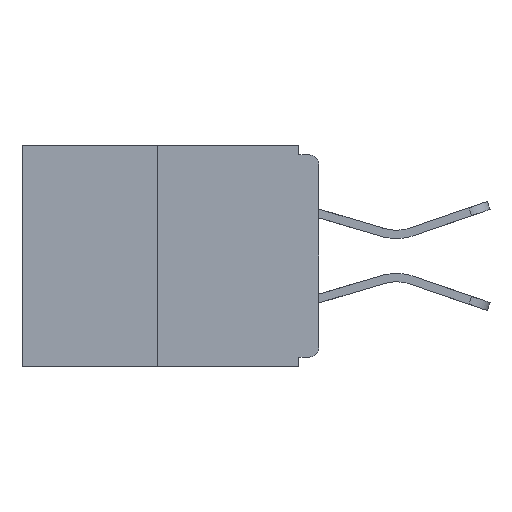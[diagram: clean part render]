
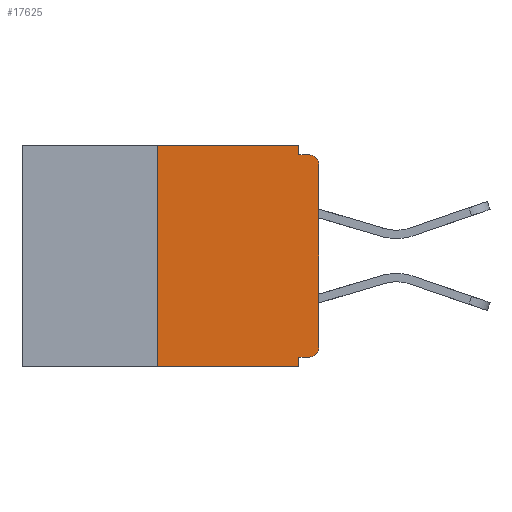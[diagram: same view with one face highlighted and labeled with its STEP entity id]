
A CAD part, left-side view. The second image highlights one B-rep face of the part: STEP entity #17625.
In plain terms, the highlighted planar face has unit normal (-1, 0, 0).
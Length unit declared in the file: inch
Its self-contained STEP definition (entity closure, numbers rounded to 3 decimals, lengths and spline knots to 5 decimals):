
#193 = VECTOR ( 'NONE', #14481, 39.37008 ) ;
#308 = DIRECTION ( 'NONE',  ( 0., 0., -1. ) ) ;
#543 = EDGE_CURVE ( 'NONE', #5200, #4194, #3123, .T. ) ;
#888 = EDGE_CURVE ( 'NONE', #13235, #17424, #23163, .T. ) ;
#1353 = CARTESIAN_POINT ( 'NONE',  ( 0., 0.031, 0. ) ) ;
#1658 = CARTESIAN_POINT ( 'NONE',  ( 0., 0.46, 0. ) ) ;
#2864 = CIRCLE ( 'NONE', #9612, 0.015 ) ;
#3123 = LINE ( 'NONE', #16304, #193 ) ;
#3310 = ORIENTED_EDGE ( 'NONE', *, *, #22976, .F. ) ;
#4194 = VERTEX_POINT ( 'NONE', #15038 ) ;
#4618 = CARTESIAN_POINT ( 'NONE',  ( 0., 0., 0. ) ) ;
#5200 = VERTEX_POINT ( 'NONE', #6665 ) ;
#5309 = VECTOR ( 'NONE', #15699, 39.37008 ) ;
#5706 = EDGE_CURVE ( 'NONE', #8212, #19450, #11725, .T. ) ;
#6344 = EDGE_CURVE ( 'NONE', #8212, #4194, #7748, .T. ) ;
#6628 = CARTESIAN_POINT ( 'NONE',  ( 0., 0., -0.328 ) ) ;
#6665 = CARTESIAN_POINT ( 'NONE',  ( 0., 0.031, -0.328 ) ) ;
#7054 = VECTOR ( 'NONE', #19556, 39.37008 ) ;
#7323 = EDGE_CURVE ( 'NONE', #19450, #19674, #19778, .T. ) ;
#7455 = CARTESIAN_POINT ( 'NONE',  ( 0., 0.031, -0.015 ) ) ;
#7739 = AXIS2_PLACEMENT_3D ( 'NONE', #13149, #18958, #15122 ) ;
#7748 = LINE ( 'NONE', #9975, #16897 ) ;
#7854 = ORIENTED_EDGE ( 'NONE', *, *, #6344, .T. ) ;
#8212 = VERTEX_POINT ( 'NONE', #15849 ) ;
#8448 = EDGE_CURVE ( 'NONE', #22660, #9009, #17925, .T. ) ;
#8456 = ORIENTED_EDGE ( 'NONE', *, *, #17105, .T. ) ;
#8824 = EDGE_CURVE ( 'NONE', #12329, #22660, #21196, .T. ) ;
#9009 = VERTEX_POINT ( 'NONE', #17903 ) ;
#9612 = AXIS2_PLACEMENT_3D ( 'NONE', #17090, #15550, #308 ) ;
#9975 = CARTESIAN_POINT ( 'NONE',  ( 0., 0.46, -0.343 ) ) ;
#10385 = DIRECTION ( 'NONE',  ( 0., 1., 0. ) ) ;
#10812 = DIRECTION ( 'NONE',  ( 0., -1., 0. ) ) ;
#10922 = ORIENTED_EDGE ( 'NONE', *, *, #7323, .F. ) ;
#11391 = FACE_OUTER_BOUND ( 'NONE', #20307, .T. ) ;
#11452 = PLANE ( 'NONE',  #7739 ) ;
#11725 = LINE ( 'NONE', #23120, #7054 ) ;
#11964 = DIRECTION ( 'NONE',  ( 0., -1., 0. ) ) ;
#12041 = ORIENTED_EDGE ( 'NONE', *, *, #543, .F. ) ;
#12329 = VERTEX_POINT ( 'NONE', #19905 ) ;
#13149 = CARTESIAN_POINT ( 'NONE',  ( 0., 0.46, 0. ) ) ;
#13235 = VERTEX_POINT ( 'NONE', #7455 ) ;
#14386 = CARTESIAN_POINT ( 'NONE',  ( 0., 0.015, -0.015 ) ) ;
#14481 = DIRECTION ( 'NONE',  ( 0., 0., -1. ) ) ;
#15038 = CARTESIAN_POINT ( 'NONE',  ( 0., 0.031, -0.343 ) ) ;
#15122 = DIRECTION ( 'NONE',  ( 0., 0., -1. ) ) ;
#15478 = ORIENTED_EDGE ( 'NONE', *, *, #8448, .T. ) ;
#15550 = DIRECTION ( 'NONE',  ( -1., 0., 0. ) ) ;
#15699 = DIRECTION ( 'NONE',  ( 0., 0., -1. ) ) ;
#15849 = CARTESIAN_POINT ( 'NONE',  ( 0., 0.25, -0.343 ) ) ;
#15937 = CARTESIAN_POINT ( 'NONE',  ( 0., 0.031, 0. ) ) ;
#16105 = VECTOR ( 'NONE', #11964, 39.37008 ) ;
#16304 = CARTESIAN_POINT ( 'NONE',  ( 0., 0.031, -0.343 ) ) ;
#16751 = LINE ( 'NONE', #15937, #5309 ) ;
#16897 = VECTOR ( 'NONE', #21461, 39.37008 ) ;
#17090 = CARTESIAN_POINT ( 'NONE',  ( 0., 0.015, -0.03 ) ) ;
#17105 = EDGE_CURVE ( 'NONE', #9009, #17424, #2864, .T. ) ;
#17332 = CARTESIAN_POINT ( 'NONE',  ( 0., 0.015, -0.313 ) ) ;
#17413 = DIRECTION ( 'NONE',  ( -1., 0., 0. ) ) ;
#17424 = VERTEX_POINT ( 'NONE', #14386 ) ;
#17602 = ORIENTED_EDGE ( 'NONE', *, *, #888, .F. ) ;
#17625 = ADVANCED_FACE ( 'NONE', ( #11391 ), #11452, .F. ) ;
#17903 = CARTESIAN_POINT ( 'NONE',  ( 0., 0., -0.03 ) ) ;
#17925 = LINE ( 'NONE', #4618, #18529 ) ;
#18529 = VECTOR ( 'NONE', #19691, 39.37008 ) ;
#18958 = DIRECTION ( 'NONE',  ( 1., 0., 0. ) ) ;
#19177 = VECTOR ( 'NONE', #10812, 39.37008 ) ;
#19237 = DIRECTION ( 'NONE',  ( 0., 0., -1. ) ) ;
#19450 = VERTEX_POINT ( 'NONE', #23061 ) ;
#19556 = DIRECTION ( 'NONE',  ( 0., 0., 1. ) ) ;
#19674 = VERTEX_POINT ( 'NONE', #1353 ) ;
#19691 = DIRECTION ( 'NONE',  ( 0., 0., 1. ) ) ;
#19778 = LINE ( 'NONE', #1658, #19177 ) ;
#19792 = CARTESIAN_POINT ( 'NONE',  ( 0., 0., -0.015 ) ) ;
#19905 = CARTESIAN_POINT ( 'NONE',  ( 0., 0.015, -0.328 ) ) ;
#20307 = EDGE_LOOP ( 'NONE', ( #10922, #22614, #7854, #12041, #23509, #21224, #15478, #8456, #17602, #3310 ) ) ;
#20331 = EDGE_CURVE ( 'NONE', #12329, #5200, #22822, .T. ) ;
#21196 = CIRCLE ( 'NONE', #21814, 0.015 ) ;
#21224 = ORIENTED_EDGE ( 'NONE', *, *, #8824, .T. ) ;
#21461 = DIRECTION ( 'NONE',  ( 0., -1., 0. ) ) ;
#21814 = AXIS2_PLACEMENT_3D ( 'NONE', #17332, #17413, #19237 ) ;
#22298 = CARTESIAN_POINT ( 'NONE',  ( 0., 0., -0.313 ) ) ;
#22614 = ORIENTED_EDGE ( 'NONE', *, *, #5706, .F. ) ;
#22660 = VERTEX_POINT ( 'NONE', #22298 ) ;
#22822 = LINE ( 'NONE', #6628, #23415 ) ;
#22976 = EDGE_CURVE ( 'NONE', #19674, #13235, #16751, .T. ) ;
#23061 = CARTESIAN_POINT ( 'NONE',  ( 0., 0.25, 0. ) ) ;
#23120 = CARTESIAN_POINT ( 'NONE',  ( 0., 0.25, 0. ) ) ;
#23163 = LINE ( 'NONE', #19792, #16105 ) ;
#23415 = VECTOR ( 'NONE', #10385, 39.37008 ) ;
#23509 = ORIENTED_EDGE ( 'NONE', *, *, #20331, .F. ) ;
